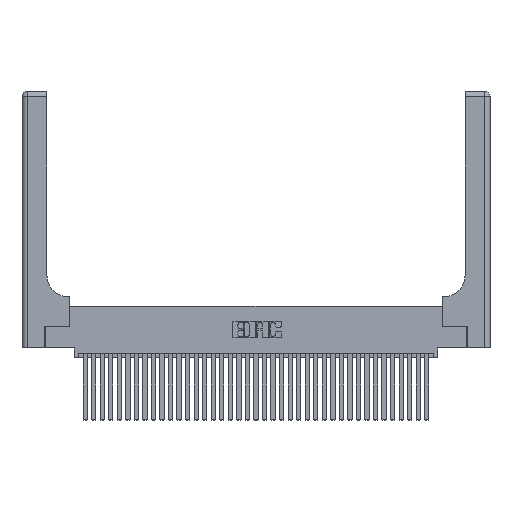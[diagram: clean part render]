
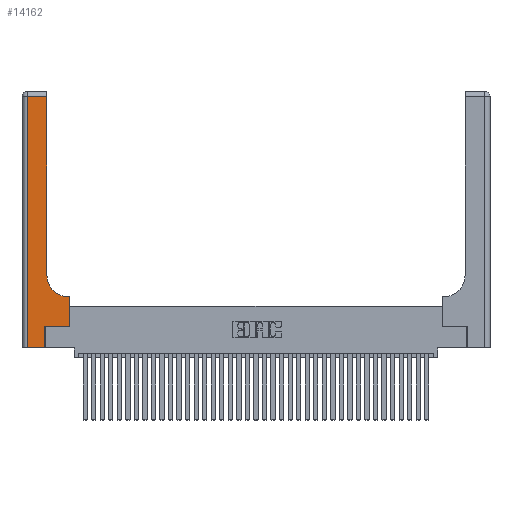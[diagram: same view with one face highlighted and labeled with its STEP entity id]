
A CAD part, top view. The second image highlights one B-rep face of the part: STEP entity #14162.
In plain terms, the highlighted planar face has unit normal (0, 0, 1).
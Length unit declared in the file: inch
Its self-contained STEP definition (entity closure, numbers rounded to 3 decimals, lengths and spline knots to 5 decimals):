
#945 = CARTESIAN_POINT ( 'NONE',  ( 0.269, 0., 0.37 ) ) ;
#1355 = VECTOR ( 'NONE', #15851, 39.37008 ) ;
#1500 = DIRECTION ( 'NONE',  ( 1., 0., 0. ) ) ;
#2023 = VERTEX_POINT ( 'NONE', #24408 ) ;
#2456 = LINE ( 'NONE', #945, #16015 ) ;
#3331 = CARTESIAN_POINT ( 'NONE',  ( 0., 3., 0.37 ) ) ;
#3493 = FACE_OUTER_BOUND ( 'NONE', #25650, .T. ) ;
#4135 = DIRECTION ( 'NONE',  ( 0., -1., 0. ) ) ;
#4402 = CARTESIAN_POINT ( 'NONE',  ( 0.06, 0., 0.37 ) ) ;
#5917 = VERTEX_POINT ( 'NONE', #10892 ) ;
#6242 = PLANE ( 'NONE',  #12917 ) ;
#8089 = VECTOR ( 'NONE', #4135, 39.37008 ) ;
#8850 = ORIENTED_EDGE ( 'NONE', *, *, #31959, .T. ) ;
#9142 = DIRECTION ( 'NONE',  ( -1., 0., 0. ) ) ;
#9143 = CARTESIAN_POINT ( 'NONE',  ( 0.2915, 0.6, 0.37 ) ) ;
#9811 = ORIENTED_EDGE ( 'NONE', *, *, #18811, .T. ) ;
#9831 = CARTESIAN_POINT ( 'NONE',  ( 0.06, 3., 0.37 ) ) ;
#10100 = DIRECTION ( 'NONE',  ( 1., 0., 0. ) ) ;
#10535 = LINE ( 'NONE', #9143, #32626 ) ;
#10892 = CARTESIAN_POINT ( 'NONE',  ( 0.2915, 0.85, 0.37 ) ) ;
#12917 = AXIS2_PLACEMENT_3D ( 'NONE', #3331, #14835, #9142 ) ;
#13053 = CARTESIAN_POINT ( 'NONE',  ( 0.269, 0.25, 0.37 ) ) ;
#14145 = LINE ( 'NONE', #33158, #20877 ) ;
#14162 = ADVANCED_FACE ( 'NONE', ( #3493 ), #6242, .F. ) ;
#14835 = DIRECTION ( 'NONE',  ( 0., 0., -1. ) ) ;
#15064 = CARTESIAN_POINT ( 'NONE',  ( 0.5585, 0.25, 0.37 ) ) ;
#15181 = CARTESIAN_POINT ( 'NONE',  ( 0., 0., 0.37 ) ) ;
#15851 = DIRECTION ( 'NONE',  ( -1., 0., 0. ) ) ;
#16015 = VECTOR ( 'NONE', #27013, 39.37008 ) ;
#16064 = VERTEX_POINT ( 'NONE', #31336 ) ;
#16307 = VERTEX_POINT ( 'NONE', #29694 ) ;
#16713 = LINE ( 'NONE', #15064, #18526 ) ;
#17574 = VECTOR ( 'NONE', #21808, 39.37008 ) ;
#17643 = CIRCLE ( 'NONE', #17864, 0.25 ) ;
#17864 = AXIS2_PLACEMENT_3D ( 'NONE', #36118, #18828, #1500 ) ;
#18526 = VECTOR ( 'NONE', #35232, 39.37008 ) ;
#18811 = EDGE_CURVE ( 'NONE', #16064, #36068, #24409, .T. ) ;
#18828 = DIRECTION ( 'NONE',  ( 0., 0., -1. ) ) ;
#18948 = CARTESIAN_POINT ( 'NONE',  ( 0.2915, 3., 0.37 ) ) ;
#19269 = EDGE_CURVE ( 'NONE', #25895, #16307, #16713, .T. ) ;
#19597 = VECTOR ( 'NONE', #32444, 39.37008 ) ;
#20233 = EDGE_CURVE ( 'NONE', #36068, #36372, #24295, .T. ) ;
#20724 = ORIENTED_EDGE ( 'NONE', *, *, #33281, .T. ) ;
#20877 = VECTOR ( 'NONE', #10100, 39.37008 ) ;
#21808 = DIRECTION ( 'NONE',  ( 0., 1., 0. ) ) ;
#22902 = ORIENTED_EDGE ( 'NONE', *, *, #34126, .T. ) ;
#23272 = ORIENTED_EDGE ( 'NONE', *, *, #20233, .T. ) ;
#23717 = ORIENTED_EDGE ( 'NONE', *, *, #24506, .T. ) ;
#24295 = LINE ( 'NONE', #9831, #8089 ) ;
#24408 = CARTESIAN_POINT ( 'NONE',  ( 0.5415, 0.6, 0.37 ) ) ;
#24409 = LINE ( 'NONE', #36035, #1355 ) ;
#24506 = EDGE_CURVE ( 'NONE', #36372, #31925, #34939, .T. ) ;
#25192 = ORIENTED_EDGE ( 'NONE', *, *, #30254, .T. ) ;
#25263 = EDGE_CURVE ( 'NONE', #16307, #2023, #10535, .T. ) ;
#25650 = EDGE_LOOP ( 'NONE', ( #22902, #9811, #23272, #23717, #25192, #8850, #28000, #32400, #20724 ) ) ;
#25895 = VERTEX_POINT ( 'NONE', #26147 ) ;
#26147 = CARTESIAN_POINT ( 'NONE',  ( 0.5585, 0.25, 0.37 ) ) ;
#26443 = DIRECTION ( 'NONE',  ( -1., 0., 0. ) ) ;
#27013 = DIRECTION ( 'NONE',  ( 0., 1., 0. ) ) ;
#28000 = ORIENTED_EDGE ( 'NONE', *, *, #19269, .T. ) ;
#29694 = CARTESIAN_POINT ( 'NONE',  ( 0.5585, 0.6, 0.37 ) ) ;
#30140 = CARTESIAN_POINT ( 'NONE',  ( 0.269, 0., 0.37 ) ) ;
#30254 = EDGE_CURVE ( 'NONE', #31925, #35737, #2456, .T. ) ;
#31336 = CARTESIAN_POINT ( 'NONE',  ( 0.2915, 2.94, 0.37 ) ) ;
#31925 = VERTEX_POINT ( 'NONE', #30140 ) ;
#31959 = EDGE_CURVE ( 'NONE', #35737, #25895, #14145, .T. ) ;
#32400 = ORIENTED_EDGE ( 'NONE', *, *, #25263, .T. ) ;
#32444 = DIRECTION ( 'NONE',  ( 1., 0., 0. ) ) ;
#32626 = VECTOR ( 'NONE', #26443, 39.37008 ) ;
#32905 = LINE ( 'NONE', #18948, #17574 ) ;
#33158 = CARTESIAN_POINT ( 'NONE',  ( 0.269, 0.25, 0.37 ) ) ;
#33281 = EDGE_CURVE ( 'NONE', #2023, #5917, #17643, .T. ) ;
#34126 = EDGE_CURVE ( 'NONE', #5917, #16064, #32905, .T. ) ;
#34555 = CARTESIAN_POINT ( 'NONE',  ( 0.06, 2.94, 0.37 ) ) ;
#34939 = LINE ( 'NONE', #15181, #19597 ) ;
#35232 = DIRECTION ( 'NONE',  ( 0., 1., 0. ) ) ;
#35737 = VERTEX_POINT ( 'NONE', #13053 ) ;
#36035 = CARTESIAN_POINT ( 'NONE',  ( 0., 2.94, 0.37 ) ) ;
#36068 = VERTEX_POINT ( 'NONE', #34555 ) ;
#36118 = CARTESIAN_POINT ( 'NONE',  ( 0.5415, 0.85, 0.37 ) ) ;
#36372 = VERTEX_POINT ( 'NONE', #4402 ) ;
